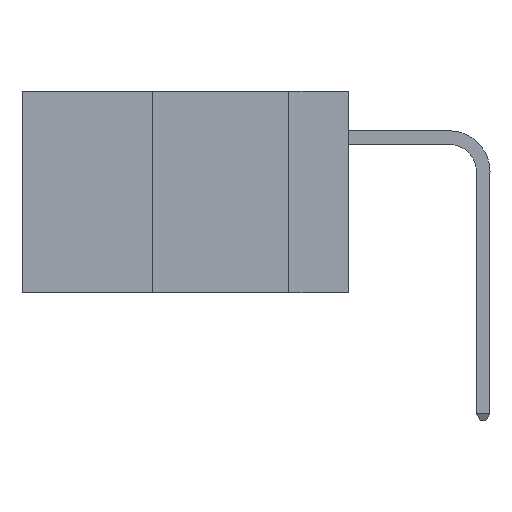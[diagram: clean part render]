
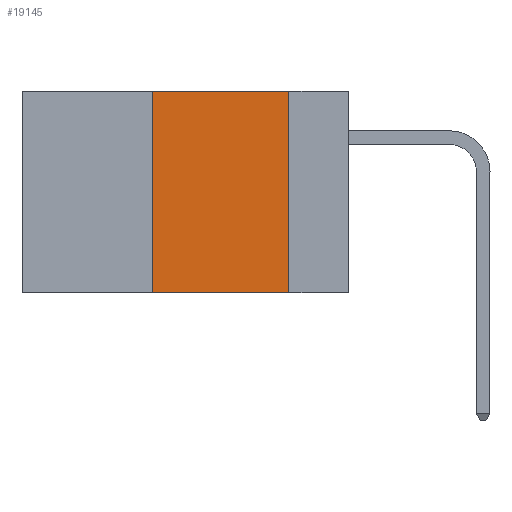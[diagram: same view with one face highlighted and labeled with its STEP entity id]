
A CAD part, left-side view. The second image highlights one B-rep face of the part: STEP entity #19145.
In plain terms, the highlighted planar face has unit normal (-1, 0, 0).
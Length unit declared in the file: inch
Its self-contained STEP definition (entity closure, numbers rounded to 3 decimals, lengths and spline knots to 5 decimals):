
#269 = CARTESIAN_POINT ( 'NONE',  ( 0., 0.11, 0. ) ) ;
#2594 = ORIENTED_EDGE ( 'NONE', *, *, #8478, .F. ) ;
#2757 = ORIENTED_EDGE ( 'NONE', *, *, #14618, .F. ) ;
#3622 = VECTOR ( 'NONE', #7582, 39.37008 ) ;
#3957 = VERTEX_POINT ( 'NONE', #22267 ) ;
#4347 = AXIS2_PLACEMENT_3D ( 'NONE', #17054, #11454, #20723 ) ;
#4438 = ORIENTED_EDGE ( 'NONE', *, *, #18795, .F. ) ;
#5054 = LINE ( 'NONE', #22604, #23698 ) ;
#5682 = CARTESIAN_POINT ( 'NONE',  ( 0., 0.6, 0. ) ) ;
#5916 = VECTOR ( 'NONE', #20957, 39.37008 ) ;
#6304 = CARTESIAN_POINT ( 'NONE',  ( 0., 0.36, -0.37 ) ) ;
#6792 = VECTOR ( 'NONE', #16099, 39.37008 ) ;
#7393 = LINE ( 'NONE', #14224, #6792 ) ;
#7582 = DIRECTION ( 'NONE',  ( 0., -1., 0. ) ) ;
#8256 = ORIENTED_EDGE ( 'NONE', *, *, #18485, .T. ) ;
#8478 = EDGE_CURVE ( 'NONE', #21348, #3957, #19152, .T. ) ;
#11454 = DIRECTION ( 'NONE',  ( 1., 0., 0. ) ) ;
#11599 = EDGE_LOOP ( 'NONE', ( #2757, #2594, #4438, #8256 ) ) ;
#12086 = VERTEX_POINT ( 'NONE', #6304 ) ;
#13405 = DIRECTION ( 'NONE',  ( 0., -1., 0. ) ) ;
#14161 = FACE_OUTER_BOUND ( 'NONE', #11599, .T. ) ;
#14224 = CARTESIAN_POINT ( 'NONE',  ( 0., 0.36, 0. ) ) ;
#14618 = EDGE_CURVE ( 'NONE', #3957, #18174, #15939, .T. ) ;
#15939 = LINE ( 'NONE', #269, #5916 ) ;
#16099 = DIRECTION ( 'NONE',  ( 0., 0., 1. ) ) ;
#17054 = CARTESIAN_POINT ( 'NONE',  ( 0., 0.6, 0. ) ) ;
#17071 = CARTESIAN_POINT ( 'NONE',  ( 0., 0.36, 0. ) ) ;
#17984 = CARTESIAN_POINT ( 'NONE',  ( 0., 0.11, -0.37 ) ) ;
#18174 = VERTEX_POINT ( 'NONE', #17984 ) ;
#18485 = EDGE_CURVE ( 'NONE', #12086, #18174, #5054, .T. ) ;
#18795 = EDGE_CURVE ( 'NONE', #12086, #21348, #7393, .T. ) ;
#18892 = PLANE ( 'NONE',  #4347 ) ;
#19145 = ADVANCED_FACE ( 'NONE', ( #14161 ), #18892, .F. ) ;
#19152 = LINE ( 'NONE', #5682, #3622 ) ;
#20723 = DIRECTION ( 'NONE',  ( 0., 0., -1. ) ) ;
#20957 = DIRECTION ( 'NONE',  ( 0., 0., -1. ) ) ;
#21348 = VERTEX_POINT ( 'NONE', #17071 ) ;
#22267 = CARTESIAN_POINT ( 'NONE',  ( 0., 0.11, 0. ) ) ;
#22604 = CARTESIAN_POINT ( 'NONE',  ( 0., 0.6, -0.37 ) ) ;
#23698 = VECTOR ( 'NONE', #13405, 39.37008 ) ;
